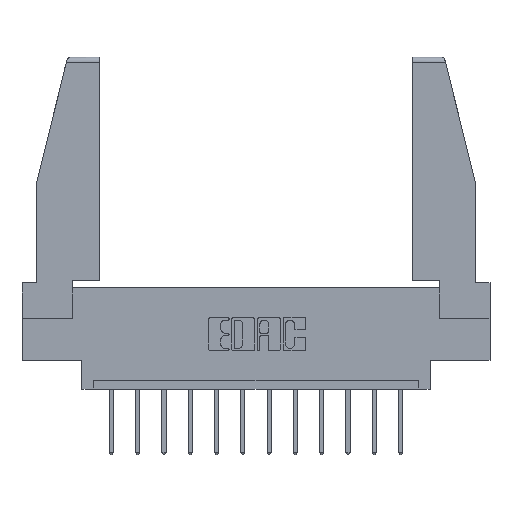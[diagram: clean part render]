
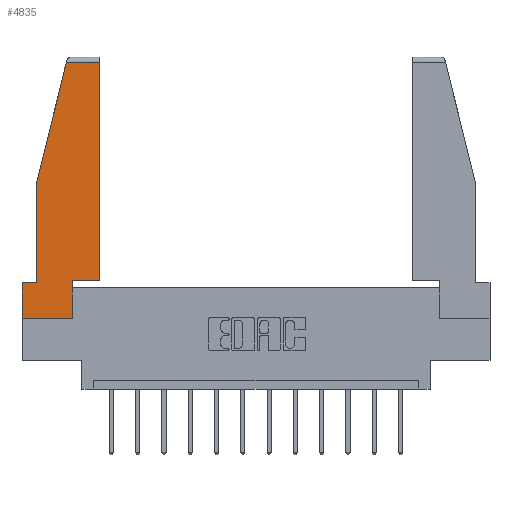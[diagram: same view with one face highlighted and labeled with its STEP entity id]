
A CAD part, top view. The second image highlights one B-rep face of the part: STEP entity #4835.
In plain terms, the highlighted planar face has unit normal (0, 0, 1).
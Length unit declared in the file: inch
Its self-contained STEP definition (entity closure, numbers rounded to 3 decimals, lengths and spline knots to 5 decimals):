
#337 = VECTOR ( 'NONE', #7547, 39.37008 ) ;
#348 = LINE ( 'NONE', #14244, #10475 ) ;
#576 = CARTESIAN_POINT ( 'NONE',  ( 0., 0.21, 0. ) ) ;
#841 = VERTEX_POINT ( 'NONE', #2590 ) ;
#1860 = CARTESIAN_POINT ( 'NONE',  ( 0.461, 1.52, 0. ) ) ;
#1905 = EDGE_CURVE ( 'NONE', #9518, #8285, #12720, .T. ) ;
#1946 = DIRECTION ( 'NONE',  ( -1., 0., 0. ) ) ;
#2224 = LINE ( 'NONE', #11577, #7664 ) ;
#2479 = ORIENTED_EDGE ( 'NONE', *, *, #2521, .T. ) ;
#2521 = EDGE_CURVE ( 'NONE', #3233, #13700, #2224, .T. ) ;
#2590 = CARTESIAN_POINT ( 'NONE',  ( 0.297, 0.223, 0. ) ) ;
#2914 = ORIENTED_EDGE ( 'NONE', *, *, #3135, .T. ) ;
#2995 = CARTESIAN_POINT ( 'NONE',  ( 0., 0.21, 0. ) ) ;
#3116 = DIRECTION ( 'NONE',  ( 0., -1., 0. ) ) ;
#3135 = EDGE_CURVE ( 'NONE', #4980, #3147, #10098, .T. ) ;
#3147 = VERTEX_POINT ( 'NONE', #6194 ) ;
#3233 = VERTEX_POINT ( 'NONE', #5388 ) ;
#3344 = LINE ( 'NONE', #10837, #8928 ) ;
#3797 = EDGE_CURVE ( 'NONE', #5630, #9518, #12460, .T. ) ;
#4063 = DIRECTION ( 'NONE',  ( 0., 0., 1. ) ) ;
#4093 = CARTESIAN_POINT ( 'NONE',  ( 0.297, 0., 0. ) ) ;
#4329 = VERTEX_POINT ( 'NONE', #4093 ) ;
#4580 = ORIENTED_EDGE ( 'NONE', *, *, #3797, .T. ) ;
#4835 = ADVANCED_FACE ( 'NONE', ( #6110 ), #5538, .T. ) ;
#4936 = CARTESIAN_POINT ( 'NONE',  ( 0.086, 0.21, 0. ) ) ;
#4980 = VERTEX_POINT ( 'NONE', #14958 ) ;
#5228 = ORIENTED_EDGE ( 'NONE', *, *, #5609, .T. ) ;
#5232 = VECTOR ( 'NONE', #1946, 39.37008 ) ;
#5388 = CARTESIAN_POINT ( 'NONE',  ( 0.461, 0.223, 0. ) ) ;
#5538 = PLANE ( 'NONE',  #10152 ) ;
#5570 = ORIENTED_EDGE ( 'NONE', *, *, #1905, .T. ) ;
#5609 = EDGE_CURVE ( 'NONE', #8285, #4329, #3344, .T. ) ;
#5630 = VERTEX_POINT ( 'NONE', #4936 ) ;
#5660 = EDGE_CURVE ( 'NONE', #841, #3233, #11839, .T. ) ;
#6110 = FACE_OUTER_BOUND ( 'NONE', #12028, .T. ) ;
#6194 = CARTESIAN_POINT ( 'NONE',  ( 0.086, 0.8, 0. ) ) ;
#6257 = VECTOR ( 'NONE', #7214, 39.37008 ) ;
#6620 = DIRECTION ( 'NONE',  ( 0., -1., 0. ) ) ;
#6813 = EDGE_CURVE ( 'NONE', #3147, #5630, #11813, .T. ) ;
#6850 = ORIENTED_EDGE ( 'NONE', *, *, #6813, .T. ) ;
#6869 = ORIENTED_EDGE ( 'NONE', *, *, #10731, .T. ) ;
#7214 = DIRECTION ( 'NONE',  ( 1., 0., 0. ) ) ;
#7547 = DIRECTION ( 'NONE',  ( -0.239, -0.971, 0. ) ) ;
#7664 = VECTOR ( 'NONE', #12707, 39.37008 ) ;
#8285 = VERTEX_POINT ( 'NONE', #9959 ) ;
#8650 = VECTOR ( 'NONE', #3116, 39.37008 ) ;
#8928 = VECTOR ( 'NONE', #10943, 39.37008 ) ;
#9050 = CARTESIAN_POINT ( 'NONE',  ( 0.086, 0.8, 0. ) ) ;
#9518 = VERTEX_POINT ( 'NONE', #12595 ) ;
#9910 = CARTESIAN_POINT ( 'NONE',  ( 0.271, 1.55, 0. ) ) ;
#9959 = CARTESIAN_POINT ( 'NONE',  ( 0., 0., 0. ) ) ;
#9990 = ORIENTED_EDGE ( 'NONE', *, *, #14657, .T. ) ;
#10098 = LINE ( 'NONE', #9910, #337 ) ;
#10152 = AXIS2_PLACEMENT_3D ( 'NONE', #10738, #4063, #10675 ) ;
#10475 = VECTOR ( 'NONE', #13073, 39.37008 ) ;
#10675 = DIRECTION ( 'NONE',  ( 1., 0., 0. ) ) ;
#10731 = EDGE_CURVE ( 'NONE', #4329, #841, #15374, .T. ) ;
#10738 = CARTESIAN_POINT ( 'NONE',  ( 0., 0., 0. ) ) ;
#10837 = CARTESIAN_POINT ( 'NONE',  ( 0., 0., 0. ) ) ;
#10943 = DIRECTION ( 'NONE',  ( 1., 0., 0. ) ) ;
#11498 = VECTOR ( 'NONE', #13299, 39.37008 ) ;
#11577 = CARTESIAN_POINT ( 'NONE',  ( 0.461, 0.223, 0. ) ) ;
#11813 = LINE ( 'NONE', #9050, #8650 ) ;
#11839 = LINE ( 'NONE', #14370, #6257 ) ;
#12023 = CARTESIAN_POINT ( 'NONE',  ( 0.297, 0., 0. ) ) ;
#12028 = EDGE_LOOP ( 'NONE', ( #2479, #9990, #2914, #6850, #4580, #5570, #5228, #6869, #13885 ) ) ;
#12460 = LINE ( 'NONE', #576, #5232 ) ;
#12595 = CARTESIAN_POINT ( 'NONE',  ( 0., 0.21, 0. ) ) ;
#12707 = DIRECTION ( 'NONE',  ( 0., 1., 0. ) ) ;
#12720 = LINE ( 'NONE', #2995, #14173 ) ;
#13073 = DIRECTION ( 'NONE',  ( -1., 0., 0. ) ) ;
#13299 = DIRECTION ( 'NONE',  ( 0., 1., 0. ) ) ;
#13700 = VERTEX_POINT ( 'NONE', #1860 ) ;
#13885 = ORIENTED_EDGE ( 'NONE', *, *, #5660, .T. ) ;
#14173 = VECTOR ( 'NONE', #6620, 39.37008 ) ;
#14244 = CARTESIAN_POINT ( 'NONE',  ( 0., 1.52, 0. ) ) ;
#14370 = CARTESIAN_POINT ( 'NONE',  ( 0.297, 0.223, 0. ) ) ;
#14657 = EDGE_CURVE ( 'NONE', #13700, #4980, #348, .T. ) ;
#14958 = CARTESIAN_POINT ( 'NONE',  ( 0.2636, 1.52, 0. ) ) ;
#15374 = LINE ( 'NONE', #12023, #11498 ) ;
